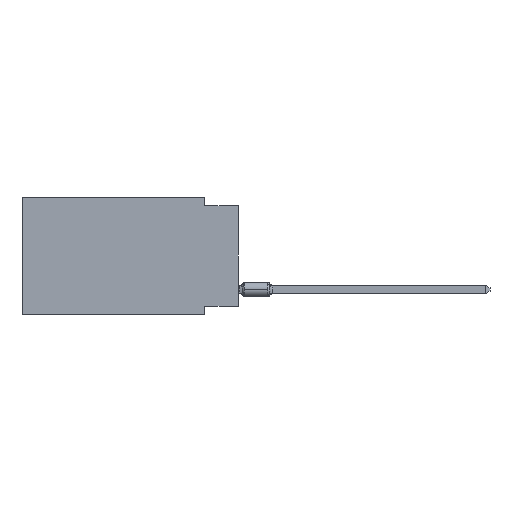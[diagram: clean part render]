
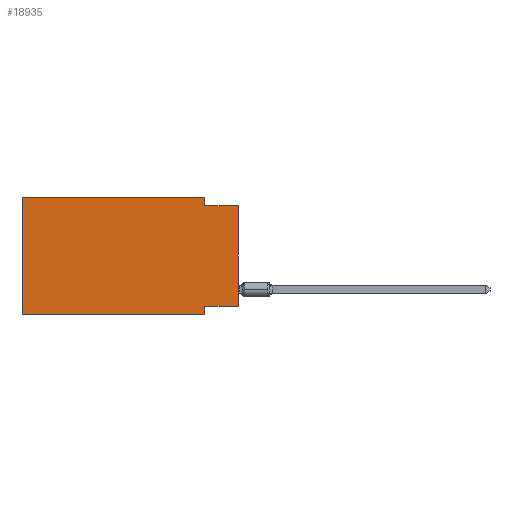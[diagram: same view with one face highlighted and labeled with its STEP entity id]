
A CAD part, left-side view. The second image highlights one B-rep face of the part: STEP entity #18935.
In plain terms, the highlighted planar face has unit normal (-1, 0, 0).
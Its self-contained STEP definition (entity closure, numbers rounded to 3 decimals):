
#304 = EDGE_CURVE ( 'NONE', #3283, #18432, #34155, .T. ) ;
#684 = LINE ( 'NONE', #30185, #18408 ) ;
#685 = ORIENTED_EDGE ( 'NONE', *, *, #1293, .F. ) ;
#1293 = EDGE_CURVE ( 'NONE', #21159, #21773, #5734, .T. ) ;
#2092 = CARTESIAN_POINT ( 'NONE',  ( 0., 2.54, -8.89 ) ) ;
#2448 = VERTEX_POINT ( 'NONE', #12959 ) ;
#3283 = VERTEX_POINT ( 'NONE', #33772 ) ;
#3511 = DIRECTION ( 'NONE',  ( 0., -1., 0. ) ) ;
#3932 = VERTEX_POINT ( 'NONE', #30858 ) ;
#4337 = DIRECTION ( 'NONE',  ( 0., 0., -1. ) ) ;
#4573 = LINE ( 'NONE', #7547, #16153 ) ;
#4692 = LINE ( 'NONE', #31586, #5198 ) ;
#4837 = LINE ( 'NONE', #20556, #6981 ) ;
#5198 = VECTOR ( 'NONE', #4337, 1000. ) ;
#5699 = ORIENTED_EDGE ( 'NONE', *, *, #23238, .F. ) ;
#5734 = LINE ( 'NONE', #11655, #32405 ) ;
#5918 = EDGE_CURVE ( 'NONE', #2448, #3932, #4573, .T. ) ;
#6117 = VECTOR ( 'NONE', #23315, 1000. ) ;
#6981 = VECTOR ( 'NONE', #25633, 1000. ) ;
#7106 = LINE ( 'NONE', #20732, #19883 ) ;
#7201 = PLANE ( 'NONE',  #23343 ) ;
#7547 = CARTESIAN_POINT ( 'NONE',  ( 0., 0., 0. ) ) ;
#7790 = ORIENTED_EDGE ( 'NONE', *, *, #12792, .F. ) ;
#8527 = DIRECTION ( 'NONE',  ( 0., 0., -1. ) ) ;
#10185 = DIRECTION ( 'NONE',  ( 1., 0., 0. ) ) ;
#10236 = CARTESIAN_POINT ( 'NONE',  ( 0., 16.383, 0. ) ) ;
#10855 = EDGE_LOOP ( 'NONE', ( #12353, #13216, #18434, #16059, #7790, #12664, #685, #5699 ) ) ;
#11655 = CARTESIAN_POINT ( 'NONE',  ( 0., 2.54, -8.89 ) ) ;
#12353 = ORIENTED_EDGE ( 'NONE', *, *, #5918, .T. ) ;
#12439 = DIRECTION ( 'NONE',  ( 0., 0., 1. ) ) ;
#12664 = ORIENTED_EDGE ( 'NONE', *, *, #20007, .T. ) ;
#12792 = EDGE_CURVE ( 'NONE', #22979, #3283, #4837, .T. ) ;
#12959 = CARTESIAN_POINT ( 'NONE',  ( 0., 0., -8.255 ) ) ;
#13216 = ORIENTED_EDGE ( 'NONE', *, *, #33544, .F. ) ;
#14301 = VERTEX_POINT ( 'NONE', #28707 ) ;
#16059 = ORIENTED_EDGE ( 'NONE', *, *, #304, .F. ) ;
#16153 = VECTOR ( 'NONE', #12439, 1000. ) ;
#16792 = LINE ( 'NONE', #19743, #21049 ) ;
#18408 = VECTOR ( 'NONE', #32462, 1000. ) ;
#18432 = VERTEX_POINT ( 'NONE', #20162 ) ;
#18434 = ORIENTED_EDGE ( 'NONE', *, *, #30354, .F. ) ;
#18935 = ADVANCED_FACE ( 'NONE', ( #26587 ), #7201, .F. ) ;
#19743 = CARTESIAN_POINT ( 'NONE',  ( 0., 0., -0.635 ) ) ;
#19883 = VECTOR ( 'NONE', #30694, 1000. ) ;
#20007 = EDGE_CURVE ( 'NONE', #22979, #21773, #684, .T. ) ;
#20162 = CARTESIAN_POINT ( 'NONE',  ( 0., 2.54, 0. ) ) ;
#20556 = CARTESIAN_POINT ( 'NONE',  ( 0., 16.383, 0. ) ) ;
#20732 = CARTESIAN_POINT ( 'NONE',  ( 0., 0., -8.255 ) ) ;
#20818 = CARTESIAN_POINT ( 'NONE',  ( 0., 16.383, 0. ) ) ;
#21049 = VECTOR ( 'NONE', #3511, 1000. ) ;
#21159 = VERTEX_POINT ( 'NONE', #23743 ) ;
#21773 = VERTEX_POINT ( 'NONE', #2092 ) ;
#22979 = VERTEX_POINT ( 'NONE', #25879 ) ;
#23238 = EDGE_CURVE ( 'NONE', #2448, #21159, #7106, .T. ) ;
#23315 = DIRECTION ( 'NONE',  ( 0., -1., 0. ) ) ;
#23343 = AXIS2_PLACEMENT_3D ( 'NONE', #20818, #10185, #23451 ) ;
#23451 = DIRECTION ( 'NONE',  ( 0., 0., -1. ) ) ;
#23743 = CARTESIAN_POINT ( 'NONE',  ( 0., 2.54, -8.255 ) ) ;
#25633 = DIRECTION ( 'NONE',  ( 0., 0., 1. ) ) ;
#25879 = CARTESIAN_POINT ( 'NONE',  ( 0., 16.383, -8.89 ) ) ;
#26587 = FACE_OUTER_BOUND ( 'NONE', #10855, .T. ) ;
#28707 = CARTESIAN_POINT ( 'NONE',  ( 0., 2.54, -0.635 ) ) ;
#30185 = CARTESIAN_POINT ( 'NONE',  ( 0., 16.383, -8.89 ) ) ;
#30354 = EDGE_CURVE ( 'NONE', #18432, #14301, #4692, .T. ) ;
#30694 = DIRECTION ( 'NONE',  ( 0., 1., 0. ) ) ;
#30858 = CARTESIAN_POINT ( 'NONE',  ( 0., 0., -0.635 ) ) ;
#31586 = CARTESIAN_POINT ( 'NONE',  ( 0., 2.54, 0. ) ) ;
#32405 = VECTOR ( 'NONE', #8527, 1000. ) ;
#32462 = DIRECTION ( 'NONE',  ( 0., -1., 0. ) ) ;
#33544 = EDGE_CURVE ( 'NONE', #14301, #3932, #16792, .T. ) ;
#33772 = CARTESIAN_POINT ( 'NONE',  ( 0., 16.383, 0. ) ) ;
#34155 = LINE ( 'NONE', #10236, #6117 ) ;
